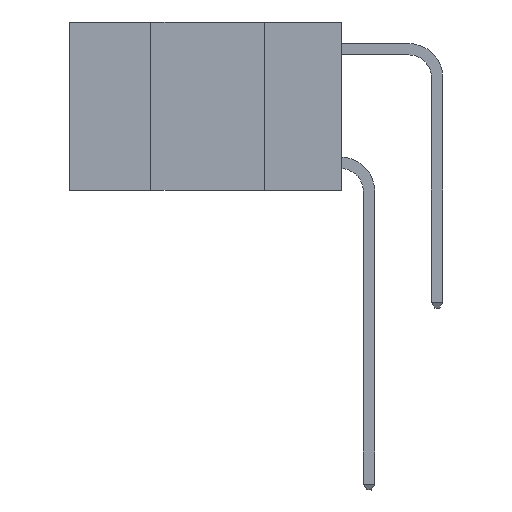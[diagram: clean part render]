
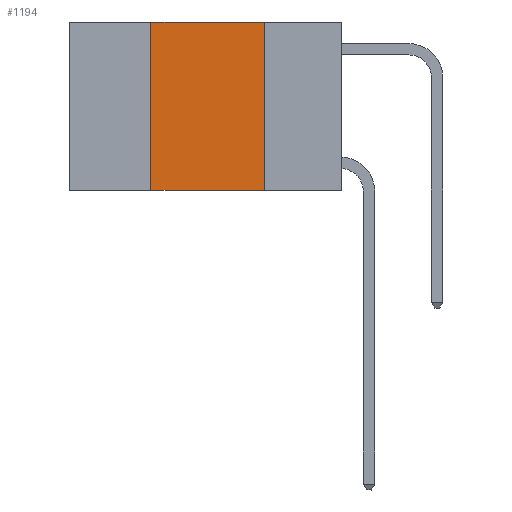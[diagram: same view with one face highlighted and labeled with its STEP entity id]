
A CAD part, left-side view. The second image highlights one B-rep face of the part: STEP entity #1194.
In plain terms, the highlighted planar face has unit normal (-1, 0, 0).
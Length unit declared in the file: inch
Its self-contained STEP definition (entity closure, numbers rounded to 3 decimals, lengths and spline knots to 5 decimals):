
#236 = CARTESIAN_POINT ( 'NONE',  ( 0., 0.42, 0. ) ) ;
#541 = VECTOR ( 'NONE', #11217, 39.37008 ) ;
#972 = EDGE_CURVE ( 'NONE', #14172, #19575, #13563, .T. ) ;
#1194 = ADVANCED_FACE ( 'NONE', ( #7806 ), #3810, .F. ) ;
#3810 = PLANE ( 'NONE',  #21677 ) ;
#5412 = DIRECTION ( 'NONE',  ( 0., 0., -1. ) ) ;
#7285 = LINE ( 'NONE', #14838, #23598 ) ;
#7559 = DIRECTION ( 'NONE',  ( 1., 0., 0. ) ) ;
#7806 = FACE_OUTER_BOUND ( 'NONE', #20442, .T. ) ;
#8251 = DIRECTION ( 'NONE',  ( 0., -1., 0. ) ) ;
#8758 = CARTESIAN_POINT ( 'NONE',  ( 0., 0.17, -0.37 ) ) ;
#8947 = ORIENTED_EDGE ( 'NONE', *, *, #9229, .F. ) ;
#9229 = EDGE_CURVE ( 'NONE', #18069, #19575, #7285, .T. ) ;
#10112 = CARTESIAN_POINT ( 'NONE',  ( 0., 0.6, -0.37 ) ) ;
#11106 = CARTESIAN_POINT ( 'NONE',  ( 0., 0.42, -0.37 ) ) ;
#11217 = DIRECTION ( 'NONE',  ( 0., -1., 0. ) ) ;
#12062 = VECTOR ( 'NONE', #20304, 39.37008 ) ;
#12211 = CARTESIAN_POINT ( 'NONE',  ( 0., 0.17, 0. ) ) ;
#13090 = LINE ( 'NONE', #20673, #541 ) ;
#13563 = LINE ( 'NONE', #10112, #24031 ) ;
#14116 = ORIENTED_EDGE ( 'NONE', *, *, #19085, .F. ) ;
#14172 = VERTEX_POINT ( 'NONE', #11106 ) ;
#14305 = ORIENTED_EDGE ( 'NONE', *, *, #972, .T. ) ;
#14838 = CARTESIAN_POINT ( 'NONE',  ( 0., 0.17, 0. ) ) ;
#18069 = VERTEX_POINT ( 'NONE', #12211 ) ;
#18381 = VERTEX_POINT ( 'NONE', #236 ) ;
#18725 = CARTESIAN_POINT ( 'NONE',  ( 0., 0.6, 0. ) ) ;
#18985 = DIRECTION ( 'NONE',  ( 0., 0., -1. ) ) ;
#19085 = EDGE_CURVE ( 'NONE', #14172, #18381, #22446, .T. ) ;
#19339 = EDGE_CURVE ( 'NONE', #18381, #18069, #13090, .T. ) ;
#19575 = VERTEX_POINT ( 'NONE', #8758 ) ;
#20304 = DIRECTION ( 'NONE',  ( 0., 0., 1. ) ) ;
#20442 = EDGE_LOOP ( 'NONE', ( #8947, #20664, #14116, #14305 ) ) ;
#20552 = CARTESIAN_POINT ( 'NONE',  ( 0., 0.42, 0. ) ) ;
#20664 = ORIENTED_EDGE ( 'NONE', *, *, #19339, .F. ) ;
#20673 = CARTESIAN_POINT ( 'NONE',  ( 0., 0.6, 0. ) ) ;
#21677 = AXIS2_PLACEMENT_3D ( 'NONE', #18725, #7559, #18985 ) ;
#22446 = LINE ( 'NONE', #20552, #12062 ) ;
#23598 = VECTOR ( 'NONE', #5412, 39.37008 ) ;
#24031 = VECTOR ( 'NONE', #8251, 39.37008 ) ;
